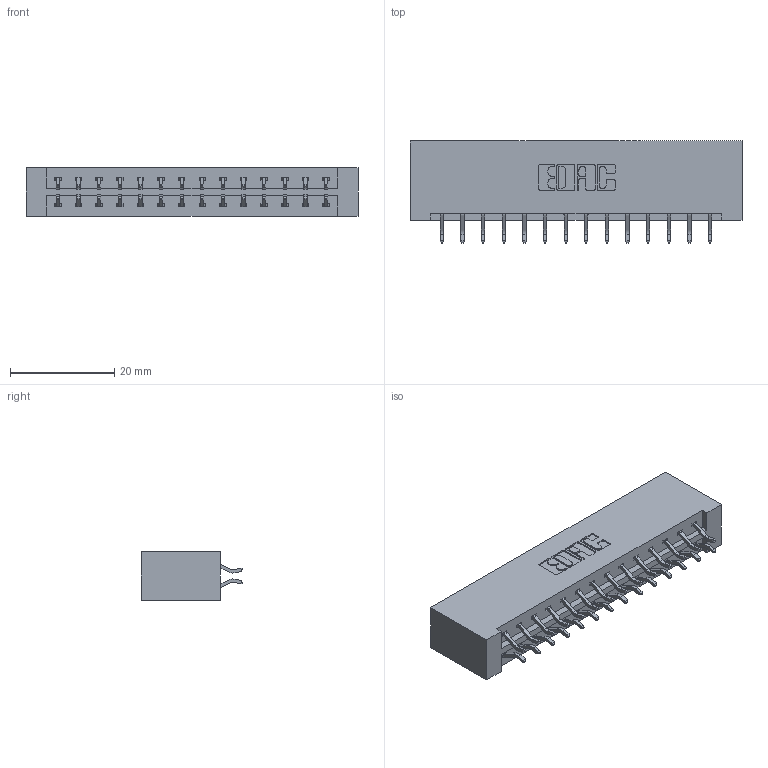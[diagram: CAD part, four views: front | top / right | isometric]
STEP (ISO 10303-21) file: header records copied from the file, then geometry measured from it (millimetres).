
FILE_DESCRIPTION (( 'STEP AP203' ), '1' );
FILE_NAME ('333-028-556-201.STEP', '2018-08-02T15:39:49', ( '' ), ( '' ), 'SwSTEP 2.0', 'SolidWorks 2016', '' );
FILE_SCHEMA (( 'CONFIG_CONTROL_DESIGN' ));
Length unit declared in the file: inch
Products named in the file (3): 333 Part_Lugless; 345-292-001_556 Tail; 333-028-556-201
Assembly tree (29 placements, depth 2):
  333-028-556-201
    333 Part_Lugless
    345-292-001_556 Tail  x28
Bounding box: 63.73 x 19.57 x 9.4 mm (x, y, z)
Volume: 6875.6 mm3; surface area: 7824.5 mm2
Topology: 29 solids, 29 shells, 1730 faces, 5131 edges, 3382 vertices
Faces by surface type: plane 1186, cylinder 544
Entity records: 12571 total; most frequent: CARTESIAN_POINT 2130, ORIENTED_EDGE 2054, DIRECTION 1851, EDGE_CURVE 1027, LINE 899, VECTOR 899, VERTEX_POINT 682, AXIS2_PLACEMENT_3D 476
